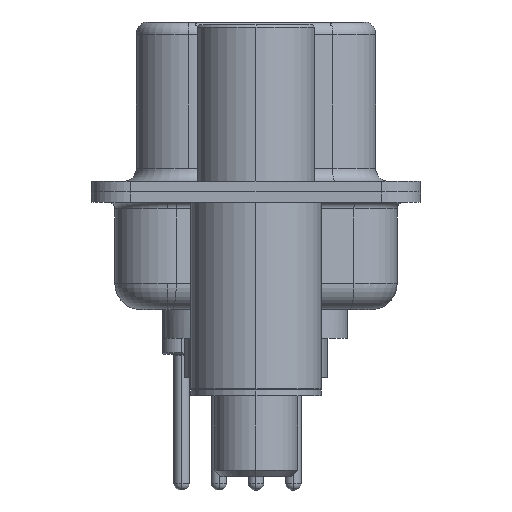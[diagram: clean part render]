
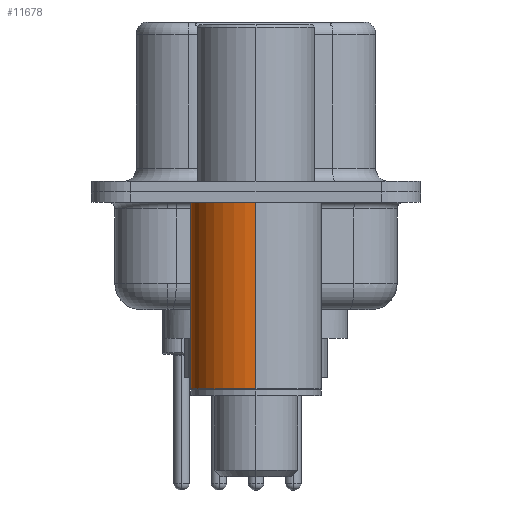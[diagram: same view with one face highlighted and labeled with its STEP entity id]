
A CAD part, left-side view. The second image highlights one B-rep face of the part: STEP entity #11678.
In plain terms, the highlighted cylindrical face has radius 2.5 mm (diameter 5 mm), a partial arc.
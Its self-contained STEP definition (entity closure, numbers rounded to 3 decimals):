
#1523 = DIRECTION ( 'NONE',  ( 0., 0., 1. ) ) ;
#2401 = DIRECTION ( 'NONE',  ( 1., 0., 0. ) ) ;
#3550 = CARTESIAN_POINT ( 'NONE',  ( -2.5, 0., -7.525 ) ) ;
#5384 = CIRCLE ( 'NONE', #9690, 2.5 ) ;
#5770 = VERTEX_POINT ( 'NONE', #7771 ) ;
#5849 = DIRECTION ( 'NONE',  ( 0., 0., 1. ) ) ;
#6468 = EDGE_CURVE ( 'NONE', #16576, #12025, #20775, .T. ) ;
#6715 = LINE ( 'NONE', #19094, #7265 ) ;
#7122 = DIRECTION ( 'NONE',  ( 0., 0., 1. ) ) ;
#7265 = VECTOR ( 'NONE', #7122, 1000. ) ;
#7771 = CARTESIAN_POINT ( 'NONE',  ( -2.5, 0., -0.4 ) ) ;
#8063 = CARTESIAN_POINT ( 'NONE',  ( 0., 0., -0.4 ) ) ;
#8070 = FACE_OUTER_BOUND ( 'NONE', #15469, .T. ) ;
#9690 = AXIS2_PLACEMENT_3D ( 'NONE', #11766, #1523, #13478 ) ;
#9720 = DIRECTION ( 'NONE',  ( 1., 0., 0. ) ) ;
#10651 = CARTESIAN_POINT ( 'NONE',  ( 2.5, 0., 0.581 ) ) ;
#11354 = EDGE_CURVE ( 'NONE', #16576, #17344, #5384, .T. ) ;
#11678 = ADVANCED_FACE ( 'NONE', ( #8070 ), #16616, .T. ) ;
#11766 = CARTESIAN_POINT ( 'NONE',  ( 0., 0., -7.525 ) ) ;
#11892 = CARTESIAN_POINT ( 'NONE',  ( 2.5, 0., -0.4 ) ) ;
#12025 = VERTEX_POINT ( 'NONE', #11892 ) ;
#12190 = EDGE_CURVE ( 'NONE', #17344, #5770, #6715, .T. ) ;
#13478 = DIRECTION ( 'NONE',  ( 1., 0., 0. ) ) ;
#14339 = CIRCLE ( 'NONE', #18134, 2.5 ) ;
#15469 = EDGE_LOOP ( 'NONE', ( #20403, #19074, #16652, #20122 ) ) ;
#16093 = CARTESIAN_POINT ( 'NONE',  ( 0., 0., 0.581 ) ) ;
#16195 = VECTOR ( 'NONE', #19866, 1000. ) ;
#16384 = EDGE_CURVE ( 'NONE', #12025, #5770, #14339, .T. ) ;
#16576 = VERTEX_POINT ( 'NONE', #22209 ) ;
#16616 = CYLINDRICAL_SURFACE ( 'NONE', #17363, 2.5 ) ;
#16652 = ORIENTED_EDGE ( 'NONE', *, *, #16384, .F. ) ;
#17344 = VERTEX_POINT ( 'NONE', #3550 ) ;
#17363 = AXIS2_PLACEMENT_3D ( 'NONE', #16093, #5849, #2401 ) ;
#18134 = AXIS2_PLACEMENT_3D ( 'NONE', #8063, #20012, #9720 ) ;
#19074 = ORIENTED_EDGE ( 'NONE', *, *, #12190, .T. ) ;
#19094 = CARTESIAN_POINT ( 'NONE',  ( -2.5, 0., 0.581 ) ) ;
#19866 = DIRECTION ( 'NONE',  ( 0., 0., 1. ) ) ;
#20012 = DIRECTION ( 'NONE',  ( 0., 0., 1. ) ) ;
#20122 = ORIENTED_EDGE ( 'NONE', *, *, #6468, .F. ) ;
#20403 = ORIENTED_EDGE ( 'NONE', *, *, #11354, .T. ) ;
#20775 = LINE ( 'NONE', #10651, #16195 ) ;
#22209 = CARTESIAN_POINT ( 'NONE',  ( 2.5, 0., -7.525 ) ) ;
